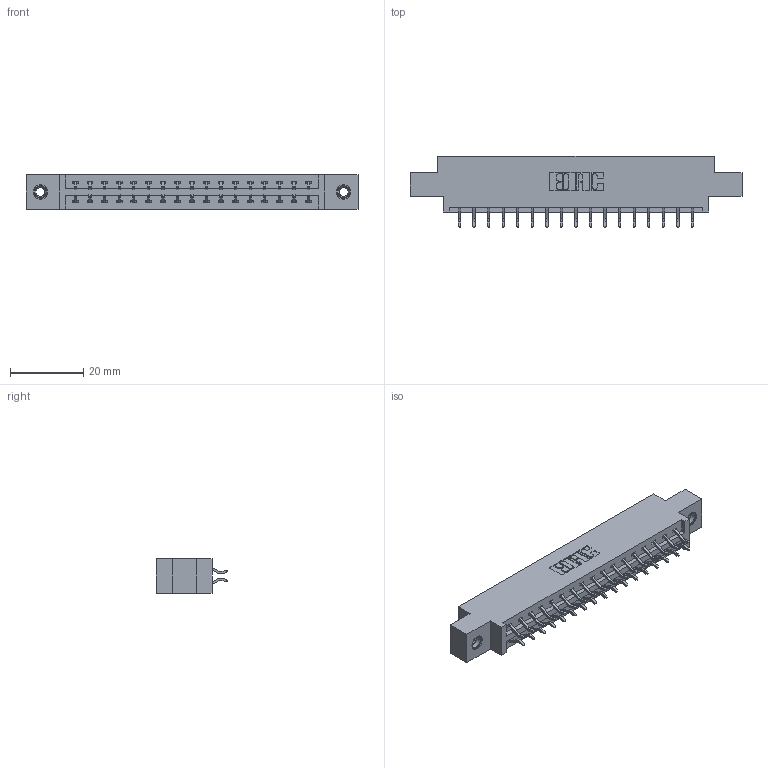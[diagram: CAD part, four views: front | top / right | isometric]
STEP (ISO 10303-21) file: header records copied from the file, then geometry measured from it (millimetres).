
FILE_DESCRIPTION (( 'STEP AP203' ), '1' );
FILE_NAME ('337-034-556-807.STEP', '2019-10-11T02:17:40', ( '' ), ( '' ), 'SwSTEP 2.0', 'SolidWorks 2016', '' );
FILE_SCHEMA (( 'CONFIG_CONTROL_DESIGN' ));
Length unit declared in the file: inch
Products named in the file (4): 345-292-001_556 Tail; 337 Part_0.170 Offset - 0.156 Dia-TI; 337-034-556-807; 345-250-001_345-250-005-103
Assembly tree (37 placements, depth 2):
  337-034-556-807
    337 Part_0.170 Offset - 0.156 Dia-TI
    345-292-001_556 Tail  x34
    345-250-001_345-250-005-103  x2
Bounding box: 90.37 x 19.57 x 9.4 mm (x, y, z)
Volume: 9059.1 mm3; surface area: 10106.4 mm2
Topology: 37 solids, 37 shells, 2218 faces, 6545 edges, 4310 vertices
Faces by surface type: plane 1534, cylinder 668, cone 12, torus 4
Entity records: 17952 total; most frequent: CARTESIAN_POINT 3041, ORIENTED_EDGE 2958, DIRECTION 2653, EDGE_CURVE 1479, LINE 1323, VECTOR 1323, VERTEX_POINT 980, AXIS2_PLACEMENT_3D 665
